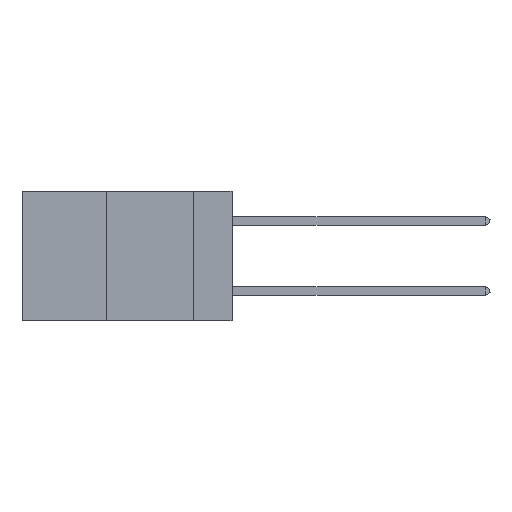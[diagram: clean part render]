
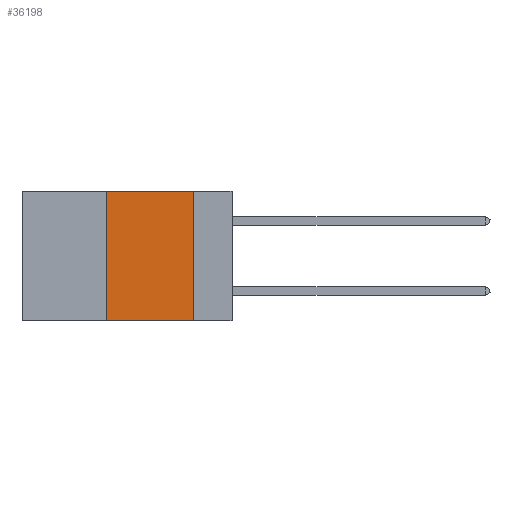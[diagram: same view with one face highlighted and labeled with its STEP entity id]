
A CAD part, left-side view. The second image highlights one B-rep face of the part: STEP entity #36198.
In plain terms, the highlighted planar face has unit normal (-1, 0, 0).
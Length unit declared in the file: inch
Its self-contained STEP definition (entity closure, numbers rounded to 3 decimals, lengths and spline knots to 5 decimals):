
#1165 = CARTESIAN_POINT ( 'NONE',  ( 0., 0.6, 0. ) ) ;
#2737 = EDGE_CURVE ( 'NONE', #26339, #12792, #14285, .T. ) ;
#3090 = VECTOR ( 'NONE', #10755, 39.37008 ) ;
#3440 = CARTESIAN_POINT ( 'NONE',  ( 0., 0.36, -0.37 ) ) ;
#3841 = LINE ( 'NONE', #37332, #26476 ) ;
#3878 = ORIENTED_EDGE ( 'NONE', *, *, #7452, .F. ) ;
#4339 = CARTESIAN_POINT ( 'NONE',  ( 0., 0.11, 0. ) ) ;
#5380 = DIRECTION ( 'NONE',  ( 1., 0., 0. ) ) ;
#7170 = VECTOR ( 'NONE', #11374, 39.37008 ) ;
#7452 = EDGE_CURVE ( 'NONE', #26339, #9406, #3841, .T. ) ;
#7972 = ORIENTED_EDGE ( 'NONE', *, *, #29211, .F. ) ;
#8222 = CARTESIAN_POINT ( 'NONE',  ( 0., 0.36, 0. ) ) ;
#8885 = CARTESIAN_POINT ( 'NONE',  ( 0., 0.11, 0. ) ) ;
#9406 = VERTEX_POINT ( 'NONE', #8222 ) ;
#9815 = ORIENTED_EDGE ( 'NONE', *, *, #2737, .T. ) ;
#10554 = LINE ( 'NONE', #4339, #13070 ) ;
#10755 = DIRECTION ( 'NONE',  ( 0., -1., 0. ) ) ;
#11374 = DIRECTION ( 'NONE',  ( 0., -1., 0. ) ) ;
#12286 = VERTEX_POINT ( 'NONE', #8885 ) ;
#12792 = VERTEX_POINT ( 'NONE', #24418 ) ;
#13070 = VECTOR ( 'NONE', #37171, 39.37008 ) ;
#14285 = LINE ( 'NONE', #36882, #7170 ) ;
#14704 = CARTESIAN_POINT ( 'NONE',  ( 0., 0.6, 0. ) ) ;
#15767 = EDGE_CURVE ( 'NONE', #9406, #12286, #27681, .T. ) ;
#21017 = PLANE ( 'NONE',  #30019 ) ;
#24334 = DIRECTION ( 'NONE',  ( 0., 0., 1. ) ) ;
#24418 = CARTESIAN_POINT ( 'NONE',  ( 0., 0.11, -0.37 ) ) ;
#26339 = VERTEX_POINT ( 'NONE', #3440 ) ;
#26476 = VECTOR ( 'NONE', #24334, 39.37008 ) ;
#27482 = FACE_OUTER_BOUND ( 'NONE', #31627, .T. ) ;
#27681 = LINE ( 'NONE', #1165, #3090 ) ;
#29211 = EDGE_CURVE ( 'NONE', #12286, #12792, #10554, .T. ) ;
#30019 = AXIS2_PLACEMENT_3D ( 'NONE', #14704, #5380, #34002 ) ;
#31627 = EDGE_LOOP ( 'NONE', ( #7972, #41193, #3878, #9815 ) ) ;
#34002 = DIRECTION ( 'NONE',  ( 0., 0., -1. ) ) ;
#36198 = ADVANCED_FACE ( 'NONE', ( #27482 ), #21017, .F. ) ;
#36882 = CARTESIAN_POINT ( 'NONE',  ( 0., 0.6, -0.37 ) ) ;
#37171 = DIRECTION ( 'NONE',  ( 0., 0., -1. ) ) ;
#37332 = CARTESIAN_POINT ( 'NONE',  ( 0., 0.36, 0. ) ) ;
#41193 = ORIENTED_EDGE ( 'NONE', *, *, #15767, .F. ) ;
